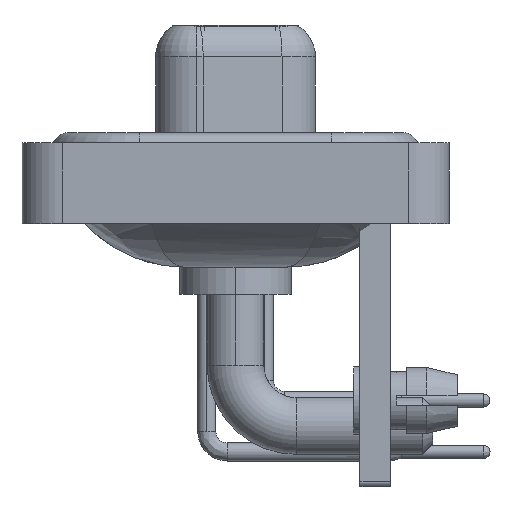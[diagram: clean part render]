
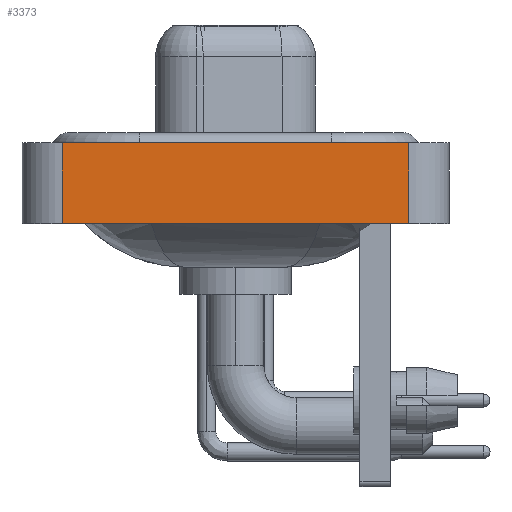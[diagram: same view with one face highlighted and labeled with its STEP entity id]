
A CAD part, left-side view. The second image highlights one B-rep face of the part: STEP entity #3373.
In plain terms, the highlighted planar face has unit normal (-1, 0, 0).
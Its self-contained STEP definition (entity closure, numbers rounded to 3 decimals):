
#975 = EDGE_CURVE ( 'NONE', #12174, #7735, #6074, .T. ) ;
#996 = VECTOR ( 'NONE', #17989, 1000. ) ;
#1069 = CARTESIAN_POINT ( 'NONE',  ( -7.35, -8.55, -3.6 ) ) ;
#1980 = DIRECTION ( 'NONE',  ( 0., -1., 0. ) ) ;
#2115 = CARTESIAN_POINT ( 'NONE',  ( -7.35, -8.55, -3.6 ) ) ;
#2713 = PLANE ( 'NONE',  #15879 ) ;
#3373 = ADVANCED_FACE ( 'NONE', ( #11465 ), #2713, .T. ) ;
#6074 = LINE ( 'NONE', #20748, #27112 ) ;
#7735 = VERTEX_POINT ( 'NONE', #21870 ) ;
#8318 = ORIENTED_EDGE ( 'NONE', *, *, #11417, .T. ) ;
#8828 = VECTOR ( 'NONE', #23161, 1000. ) ;
#9491 = DIRECTION ( 'NONE',  ( 0., 0., 1. ) ) ;
#10549 = VERTEX_POINT ( 'NONE', #2115 ) ;
#11417 = EDGE_CURVE ( 'NONE', #16131, #10549, #25365, .T. ) ;
#11419 = LINE ( 'NONE', #15684, #996 ) ;
#11465 = FACE_OUTER_BOUND ( 'NONE', #20503, .T. ) ;
#12174 = VERTEX_POINT ( 'NONE', #13829 ) ;
#13829 = CARTESIAN_POINT ( 'NONE',  ( -7.35, 8.55, 0.4 ) ) ;
#15607 = DIRECTION ( 'NONE',  ( 0., 0., 1. ) ) ;
#15684 = CARTESIAN_POINT ( 'NONE',  ( -7.35, 8.55, -3.6 ) ) ;
#15733 = DIRECTION ( 'NONE',  ( -1., 0., 0. ) ) ;
#15879 = AXIS2_PLACEMENT_3D ( 'NONE', #1069, #15733, #15607 ) ;
#16131 = VERTEX_POINT ( 'NONE', #24997 ) ;
#17088 = ORIENTED_EDGE ( 'NONE', *, *, #975, .F. ) ;
#17989 = DIRECTION ( 'NONE',  ( 0., 0., 1. ) ) ;
#19288 = VECTOR ( 'NONE', #9491, 1000. ) ;
#19441 = ORIENTED_EDGE ( 'NONE', *, *, #20527, .F. ) ;
#19580 = ORIENTED_EDGE ( 'NONE', *, *, #21849, .T. ) ;
#19939 = LINE ( 'NONE', #26521, #19288 ) ;
#20503 = EDGE_LOOP ( 'NONE', ( #19580, #17088, #19441, #8318 ) ) ;
#20527 = EDGE_CURVE ( 'NONE', #16131, #12174, #11419, .T. ) ;
#20748 = CARTESIAN_POINT ( 'NONE',  ( -7.35, -8.55, 0.4 ) ) ;
#21849 = EDGE_CURVE ( 'NONE', #10549, #7735, #19939, .T. ) ;
#21870 = CARTESIAN_POINT ( 'NONE',  ( -7.35, -8.55, 0.4 ) ) ;
#23161 = DIRECTION ( 'NONE',  ( 0., -1., 0. ) ) ;
#23299 = CARTESIAN_POINT ( 'NONE',  ( -7.35, -8.55, -3.6 ) ) ;
#24997 = CARTESIAN_POINT ( 'NONE',  ( -7.35, 8.55, -3.6 ) ) ;
#25365 = LINE ( 'NONE', #23299, #8828 ) ;
#26521 = CARTESIAN_POINT ( 'NONE',  ( -7.35, -8.55, -3.6 ) ) ;
#27112 = VECTOR ( 'NONE', #1980, 1000. ) ;
